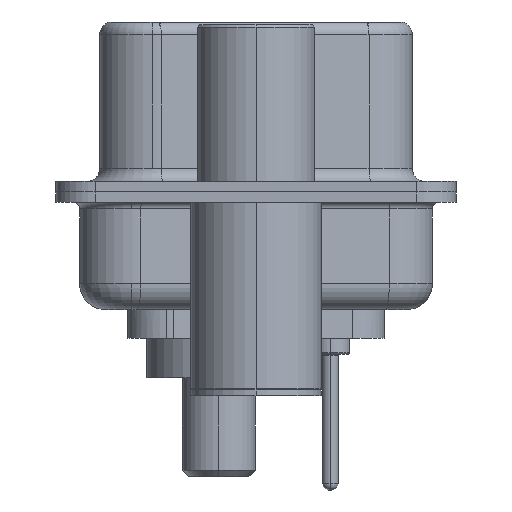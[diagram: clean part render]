
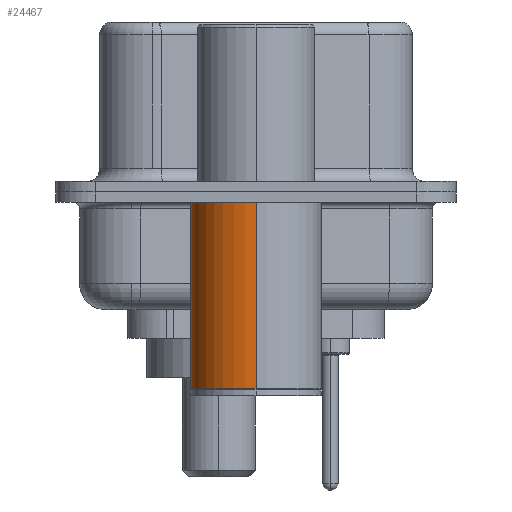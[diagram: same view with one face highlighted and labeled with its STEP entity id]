
A CAD part, left-side view. The second image highlights one B-rep face of the part: STEP entity #24467.
In plain terms, the highlighted cylindrical face has radius 2.5 mm (diameter 5 mm), a partial arc.
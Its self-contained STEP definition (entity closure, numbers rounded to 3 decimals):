
#91 = ORIENTED_EDGE ( 'NONE', *, *, #15790, .T. ) ;
#450 = CARTESIAN_POINT ( 'NONE',  ( 2.5, 0., -0.4 ) ) ;
#485 = CARTESIAN_POINT ( 'NONE',  ( -2.5, 0., -7.525 ) ) ;
#954 = EDGE_LOOP ( 'NONE', ( #23881, #91, #21318, #12879 ) ) ;
#1532 = VERTEX_POINT ( 'NONE', #450 ) ;
#2024 = LINE ( 'NONE', #27942, #12945 ) ;
#4605 = CARTESIAN_POINT ( 'NONE',  ( 0., 0., -7.525 ) ) ;
#4621 = VERTEX_POINT ( 'NONE', #485 ) ;
#5647 = CIRCLE ( 'NONE', #26147, 2.5 ) ;
#6835 = DIRECTION ( 'NONE',  ( 1., 0., 0. ) ) ;
#6836 = DIRECTION ( 'NONE',  ( 0., 0., 1. ) ) ;
#6943 = FACE_OUTER_BOUND ( 'NONE', #954, .T. ) ;
#9076 = EDGE_CURVE ( 'NONE', #16953, #1532, #13118, .T. ) ;
#9781 = DIRECTION ( 'NONE',  ( 0., 0., 1. ) ) ;
#11865 = VERTEX_POINT ( 'NONE', #17103 ) ;
#11965 = CIRCLE ( 'NONE', #19858, 2.5 ) ;
#12879 = ORIENTED_EDGE ( 'NONE', *, *, #9076, .F. ) ;
#12945 = VECTOR ( 'NONE', #23572, 1000. ) ;
#13118 = LINE ( 'NONE', #22056, #24756 ) ;
#15790 = EDGE_CURVE ( 'NONE', #4621, #11865, #2024, .T. ) ;
#16953 = VERTEX_POINT ( 'NONE', #17524 ) ;
#17101 = CYLINDRICAL_SURFACE ( 'NONE', #21308, 2.5 ) ;
#17103 = CARTESIAN_POINT ( 'NONE',  ( -2.5, 0., -0.4 ) ) ;
#17524 = CARTESIAN_POINT ( 'NONE',  ( 2.5, 0., -7.525 ) ) ;
#17550 = DIRECTION ( 'NONE',  ( 0., 0., 1. ) ) ;
#19813 = DIRECTION ( 'NONE',  ( 0., 0., 1. ) ) ;
#19858 = AXIS2_PLACEMENT_3D ( 'NONE', #22862, #9781, #25055 ) ;
#21308 = AXIS2_PLACEMENT_3D ( 'NONE', #26092, #17550, #21980 ) ;
#21318 = ORIENTED_EDGE ( 'NONE', *, *, #26613, .F. ) ;
#21980 = DIRECTION ( 'NONE',  ( 1., 0., 0. ) ) ;
#22056 = CARTESIAN_POINT ( 'NONE',  ( 2.5, 0., 0.581 ) ) ;
#22596 = EDGE_CURVE ( 'NONE', #16953, #4621, #5647, .T. ) ;
#22862 = CARTESIAN_POINT ( 'NONE',  ( 0., 0., -0.4 ) ) ;
#23572 = DIRECTION ( 'NONE',  ( 0., 0., 1. ) ) ;
#23881 = ORIENTED_EDGE ( 'NONE', *, *, #22596, .T. ) ;
#24467 = ADVANCED_FACE ( 'NONE', ( #6943 ), #17101, .T. ) ;
#24756 = VECTOR ( 'NONE', #6836, 1000. ) ;
#25055 = DIRECTION ( 'NONE',  ( 1., 0., 0. ) ) ;
#26092 = CARTESIAN_POINT ( 'NONE',  ( 0., 0., 0.581 ) ) ;
#26147 = AXIS2_PLACEMENT_3D ( 'NONE', #4605, #19813, #6835 ) ;
#26613 = EDGE_CURVE ( 'NONE', #1532, #11865, #11965, .T. ) ;
#27942 = CARTESIAN_POINT ( 'NONE',  ( -2.5, 0., 0.581 ) ) ;
